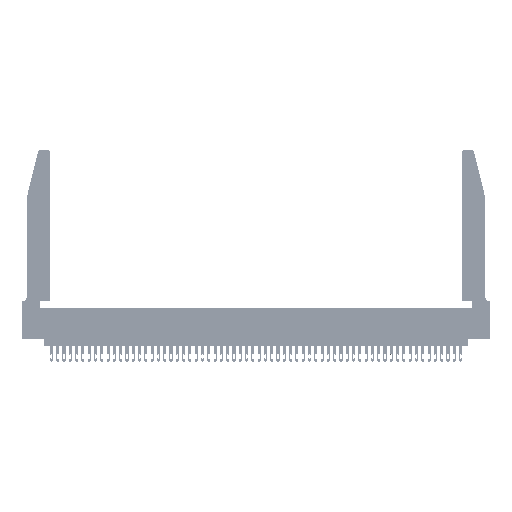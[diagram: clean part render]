
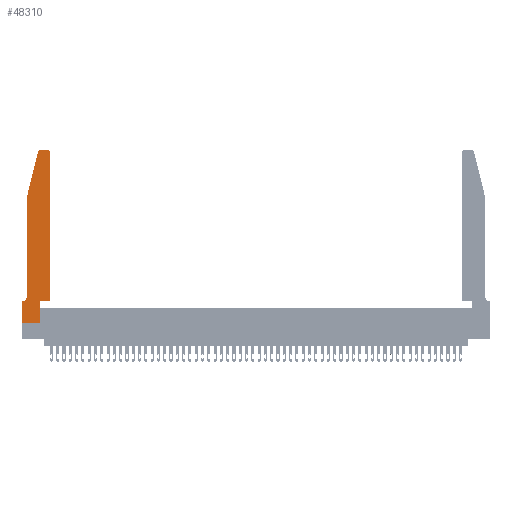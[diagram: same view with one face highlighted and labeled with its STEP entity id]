
A CAD part, top view. The second image highlights one B-rep face of the part: STEP entity #48310.
In plain terms, the highlighted planar face has unit normal (0, 0, 1).
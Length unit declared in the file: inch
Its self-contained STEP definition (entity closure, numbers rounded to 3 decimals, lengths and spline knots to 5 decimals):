
#2137 = ORIENTED_EDGE ( 'NONE', *, *, #43849, .T. ) ;
#3144 = CIRCLE ( 'NONE', #35077, 0.03 ) ;
#4133 = DIRECTION ( 'NONE',  ( 0., -1., 0. ) ) ;
#4614 = DIRECTION ( 'NONE',  ( 1., 0., 0. ) ) ;
#5094 = VERTEX_POINT ( 'NONE', #13748 ) ;
#5245 = DIRECTION ( 'NONE',  ( 0., 1., 0. ) ) ;
#5256 = CARTESIAN_POINT ( 'NONE',  ( 0.4505, 0.35, 0.37 ) ) ;
#5339 = VERTEX_POINT ( 'NONE', #40762 ) ;
#5565 = CARTESIAN_POINT ( 'NONE',  ( 0.4505, 2.72, 0.37 ) ) ;
#5670 = EDGE_CURVE ( 'NONE', #31265, #49005, #31331, .T. ) ;
#6784 = CARTESIAN_POINT ( 'NONE',  ( 0.0055, 0.42, 0.37 ) ) ;
#6923 = VECTOR ( 'NONE', #9151, 39.37008 ) ;
#7832 = ORIENTED_EDGE ( 'NONE', *, *, #9641, .T. ) ;
#8142 = LINE ( 'NONE', #49364, #9456 ) ;
#9057 = CARTESIAN_POINT ( 'NONE',  ( 0.0755, 2., 0.37 ) ) ;
#9151 = DIRECTION ( 'NONE',  ( 1., 0., 0. ) ) ;
#9170 = CARTESIAN_POINT ( 'NONE',  ( 0.2865, 0.35, 0.37 ) ) ;
#9338 = CARTESIAN_POINT ( 'NONE',  ( 0.2865, 0.35, 0.37 ) ) ;
#9456 = VECTOR ( 'NONE', #4133, 39.37008 ) ;
#9641 = EDGE_CURVE ( 'NONE', #18513, #16109, #3144, .T. ) ;
#9912 = VECTOR ( 'NONE', #14358, 39.37008 ) ;
#10005 = CARTESIAN_POINT ( 'NONE',  ( 0.4205, 2.72, 0.37 ) ) ;
#10387 = CARTESIAN_POINT ( 'NONE',  ( 0.0755, 2., 0.37 ) ) ;
#11450 = DIRECTION ( 'NONE',  ( 0., 0., -1. ) ) ;
#11900 = LINE ( 'NONE', #45760, #42219 ) ;
#12073 = CARTESIAN_POINT ( 'NONE',  ( 0., 0.35, 0.37 ) ) ;
#12407 = ORIENTED_EDGE ( 'NONE', *, *, #29660, .T. ) ;
#12420 = DIRECTION ( 'NONE',  ( 0., -1., 0. ) ) ;
#12901 = EDGE_CURVE ( 'NONE', #16109, #32896, #29284, .T. ) ;
#13017 = ORIENTED_EDGE ( 'NONE', *, *, #32012, .T. ) ;
#13748 = CARTESIAN_POINT ( 'NONE',  ( 0.4505, 0.35, 0.37 ) ) ;
#14358 = DIRECTION ( 'NONE',  ( -0.239, -0.971, 0. ) ) ;
#14580 = VERTEX_POINT ( 'NONE', #37161 ) ;
#14863 = CARTESIAN_POINT ( 'NONE',  ( 0.25487, 2.72718, 0.37 ) ) ;
#15547 = EDGE_CURVE ( 'NONE', #45590, #30370, #34074, .T. ) ;
#16109 = VERTEX_POINT ( 'NONE', #14863 ) ;
#17097 = CARTESIAN_POINT ( 'NONE',  ( 0., 0., 0.37 ) ) ;
#17474 = ORIENTED_EDGE ( 'NONE', *, *, #41097, .T. ) ;
#17537 = ORIENTED_EDGE ( 'NONE', *, *, #34448, .T. ) ;
#18428 = DIRECTION ( 'NONE',  ( 1., 0., 0. ) ) ;
#18513 = VERTEX_POINT ( 'NONE', #35293 ) ;
#18936 = VECTOR ( 'NONE', #30477, 39.37008 ) ;
#19023 = VERTEX_POINT ( 'NONE', #35968 ) ;
#19412 = FACE_OUTER_BOUND ( 'NONE', #26390, .T. ) ;
#22592 = PLANE ( 'NONE',  #44603 ) ;
#24132 = DIRECTION ( 'NONE',  ( -1., 0., 0. ) ) ;
#24831 = CARTESIAN_POINT ( 'NONE',  ( 0.0055, 0.35, 0.37 ) ) ;
#25320 = ORIENTED_EDGE ( 'NONE', *, *, #5670, .T. ) ;
#25876 = AXIS2_PLACEMENT_3D ( 'NONE', #10005, #47345, #48775 ) ;
#26390 = EDGE_LOOP ( 'NONE', ( #12407, #7832, #30635, #52866, #46370, #35827, #13017, #2137, #25320, #17474, #30483, #17537 ) ) ;
#27449 = EDGE_CURVE ( 'NONE', #5094, #44063, #29925, .T. ) ;
#27909 = CARTESIAN_POINT ( 'NONE',  ( 0.0755, 0.35, 0.37 ) ) ;
#28020 = CARTESIAN_POINT ( 'NONE',  ( 0.2605, 2.75, 0.37 ) ) ;
#28418 = DIRECTION ( 'NONE',  ( 0., 0., 1. ) ) ;
#29110 = EDGE_CURVE ( 'NONE', #14580, #45590, #37510, .T. ) ;
#29284 = LINE ( 'NONE', #10387, #9912 ) ;
#29660 = EDGE_CURVE ( 'NONE', #19023, #18513, #45856, .T. ) ;
#29925 = LINE ( 'NONE', #5256, #18936 ) ;
#30359 = VECTOR ( 'NONE', #40435, 39.37008 ) ;
#30370 = VERTEX_POINT ( 'NONE', #12073 ) ;
#30477 = DIRECTION ( 'NONE',  ( 0., 1., 0. ) ) ;
#30483 = ORIENTED_EDGE ( 'NONE', *, *, #27449, .T. ) ;
#30635 = ORIENTED_EDGE ( 'NONE', *, *, #12901, .T. ) ;
#31265 = VERTEX_POINT ( 'NONE', #47843 ) ;
#31331 = LINE ( 'NONE', #9170, #38420 ) ;
#32012 = EDGE_CURVE ( 'NONE', #30370, #5339, #8142, .T. ) ;
#32499 = DIRECTION ( 'NONE',  ( 1., 0., 0. ) ) ;
#32786 = VECTOR ( 'NONE', #24132, 39.37008 ) ;
#32896 = VERTEX_POINT ( 'NONE', #9057 ) ;
#33598 = VECTOR ( 'NONE', #32499, 39.37008 ) ;
#34005 = CARTESIAN_POINT ( 'NONE',  ( 0.4505, 0.35, 0.37 ) ) ;
#34074 = LINE ( 'NONE', #27909, #32786 ) ;
#34448 = EDGE_CURVE ( 'NONE', #44063, #19023, #47848, .T. ) ;
#34997 = CARTESIAN_POINT ( 'NONE',  ( 0., 0.35, 0.37 ) ) ;
#35077 = AXIS2_PLACEMENT_3D ( 'NONE', #48973, #28418, #4614 ) ;
#35170 = DIRECTION ( 'NONE',  ( 0., 0., 1. ) ) ;
#35293 = CARTESIAN_POINT ( 'NONE',  ( 0.284, 2.75, 0.37 ) ) ;
#35633 = DIRECTION ( 'NONE',  ( -1., 0., 0. ) ) ;
#35827 = ORIENTED_EDGE ( 'NONE', *, *, #15547, .T. ) ;
#35968 = CARTESIAN_POINT ( 'NONE',  ( 0.4205, 2.75, 0.37 ) ) ;
#36631 = LINE ( 'NONE', #17097, #6923 ) ;
#37161 = CARTESIAN_POINT ( 'NONE',  ( 0.0755, 0.42, 0.37 ) ) ;
#37510 = CIRCLE ( 'NONE', #46079, 0.07 ) ;
#38420 = VECTOR ( 'NONE', #5245, 39.37008 ) ;
#40435 = DIRECTION ( 'NONE',  ( -1., 0., 0. ) ) ;
#40762 = CARTESIAN_POINT ( 'NONE',  ( 0., 0., 0.37 ) ) ;
#41097 = EDGE_CURVE ( 'NONE', #49005, #5094, #46489, .T. ) ;
#42219 = VECTOR ( 'NONE', #12420, 39.37008 ) ;
#43849 = EDGE_CURVE ( 'NONE', #5339, #31265, #36631, .T. ) ;
#44063 = VERTEX_POINT ( 'NONE', #5565 ) ;
#44603 = AXIS2_PLACEMENT_3D ( 'NONE', #34997, #35170, #18428 ) ;
#45590 = VERTEX_POINT ( 'NONE', #24831 ) ;
#45760 = CARTESIAN_POINT ( 'NONE',  ( 0.0755, 2., 0.37 ) ) ;
#45856 = LINE ( 'NONE', #28020, #30359 ) ;
#46079 = AXIS2_PLACEMENT_3D ( 'NONE', #6784, #11450, #35633 ) ;
#46370 = ORIENTED_EDGE ( 'NONE', *, *, #29110, .T. ) ;
#46489 = LINE ( 'NONE', #34005, #33598 ) ;
#47345 = DIRECTION ( 'NONE',  ( 0., 0., 1. ) ) ;
#47843 = CARTESIAN_POINT ( 'NONE',  ( 0.2865, 0., 0.37 ) ) ;
#47848 = CIRCLE ( 'NONE', #25876, 0.03 ) ;
#48310 = ADVANCED_FACE ( 'NONE', ( #19412 ), #22592, .T. ) ;
#48775 = DIRECTION ( 'NONE',  ( 1., 0., 0. ) ) ;
#48973 = CARTESIAN_POINT ( 'NONE',  ( 0.284, 2.72, 0.37 ) ) ;
#49005 = VERTEX_POINT ( 'NONE', #9338 ) ;
#49364 = CARTESIAN_POINT ( 'NONE',  ( 0., 0., 0.37 ) ) ;
#51706 = EDGE_CURVE ( 'NONE', #32896, #14580, #11900, .T. ) ;
#52866 = ORIENTED_EDGE ( 'NONE', *, *, #51706, .T. ) ;
